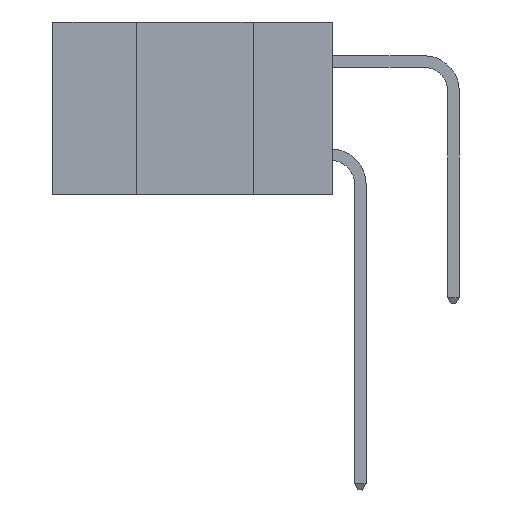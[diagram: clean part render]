
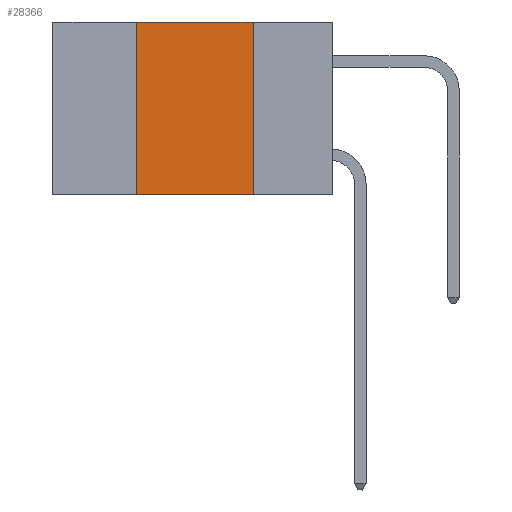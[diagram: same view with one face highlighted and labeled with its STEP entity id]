
A CAD part, left-side view. The second image highlights one B-rep face of the part: STEP entity #28366.
In plain terms, the highlighted planar face has unit normal (-1, 0, 0).
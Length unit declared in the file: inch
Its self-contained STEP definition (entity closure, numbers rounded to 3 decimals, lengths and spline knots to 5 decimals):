
#1705 = CARTESIAN_POINT ( 'NONE',  ( 0., 0.6, 0. ) ) ;
#2711 = CARTESIAN_POINT ( 'NONE',  ( 0., 0.17, 0. ) ) ;
#2908 = ORIENTED_EDGE ( 'NONE', *, *, #31445, .T. ) ;
#5734 = ORIENTED_EDGE ( 'NONE', *, *, #6581, .F. ) ;
#6581 = EDGE_CURVE ( 'NONE', #15725, #25667, #23828, .T. ) ;
#7297 = DIRECTION ( 'NONE',  ( 0., 0., 1. ) ) ;
#8490 = VERTEX_POINT ( 'NONE', #31800 ) ;
#9183 = PLANE ( 'NONE',  #11390 ) ;
#9503 = DIRECTION ( 'NONE',  ( 1., 0., 0. ) ) ;
#9944 = CARTESIAN_POINT ( 'NONE',  ( 0., 0.17, -0.37 ) ) ;
#11390 = AXIS2_PLACEMENT_3D ( 'NONE', #1705, #9503, #26773 ) ;
#13534 = EDGE_LOOP ( 'NONE', ( #26874, #5734, #30779, #2908 ) ) ;
#15725 = VERTEX_POINT ( 'NONE', #30517 ) ;
#16418 = DIRECTION ( 'NONE',  ( 0., -1., 0. ) ) ;
#17316 = VERTEX_POINT ( 'NONE', #9944 ) ;
#17725 = VECTOR ( 'NONE', #16418, 39.37008 ) ;
#18919 = DIRECTION ( 'NONE',  ( 0., -1., 0. ) ) ;
#20177 = CARTESIAN_POINT ( 'NONE',  ( 0., 0.17, 0. ) ) ;
#21627 = LINE ( 'NONE', #30054, #23994 ) ;
#23189 = VECTOR ( 'NONE', #27569, 39.37008 ) ;
#23673 = EDGE_CURVE ( 'NONE', #25667, #17316, #29863, .T. ) ;
#23828 = LINE ( 'NONE', #26291, #27352 ) ;
#23994 = VECTOR ( 'NONE', #7297, 39.37008 ) ;
#24209 = FACE_OUTER_BOUND ( 'NONE', #13534, .T. ) ;
#24441 = LINE ( 'NONE', #25992, #17725 ) ;
#25667 = VERTEX_POINT ( 'NONE', #20177 ) ;
#25992 = CARTESIAN_POINT ( 'NONE',  ( 0., 0.6, -0.37 ) ) ;
#26291 = CARTESIAN_POINT ( 'NONE',  ( 0., 0.6, 0. ) ) ;
#26773 = DIRECTION ( 'NONE',  ( 0., 0., -1. ) ) ;
#26874 = ORIENTED_EDGE ( 'NONE', *, *, #23673, .F. ) ;
#27352 = VECTOR ( 'NONE', #18919, 39.37008 ) ;
#27569 = DIRECTION ( 'NONE',  ( 0., 0., -1. ) ) ;
#28366 = ADVANCED_FACE ( 'NONE', ( #24209 ), #9183, .F. ) ;
#29863 = LINE ( 'NONE', #2711, #23189 ) ;
#30054 = CARTESIAN_POINT ( 'NONE',  ( 0., 0.42, 0. ) ) ;
#30517 = CARTESIAN_POINT ( 'NONE',  ( 0., 0.42, 0. ) ) ;
#30779 = ORIENTED_EDGE ( 'NONE', *, *, #32061, .F. ) ;
#31445 = EDGE_CURVE ( 'NONE', #8490, #17316, #24441, .T. ) ;
#31800 = CARTESIAN_POINT ( 'NONE',  ( 0., 0.42, -0.37 ) ) ;
#32061 = EDGE_CURVE ( 'NONE', #8490, #15725, #21627, .T. ) ;
